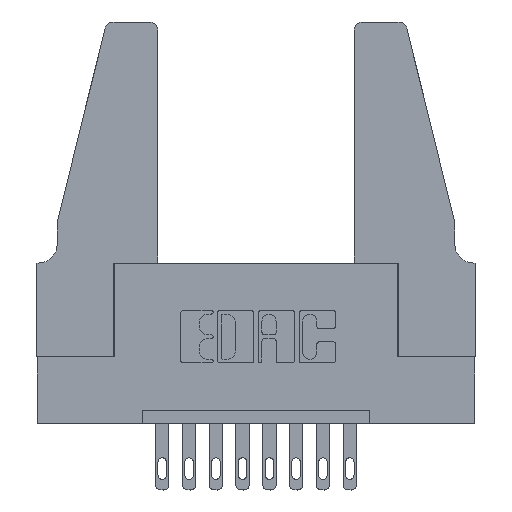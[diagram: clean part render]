
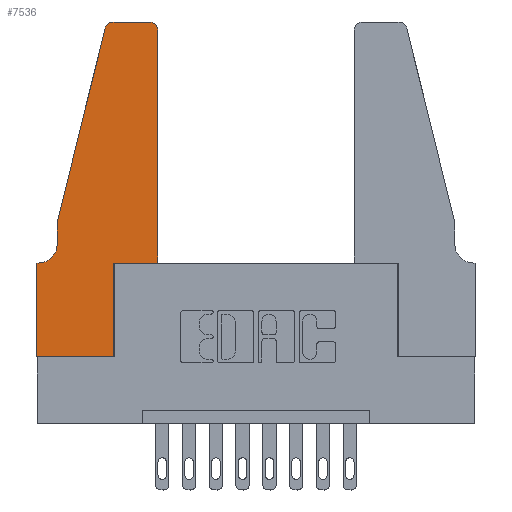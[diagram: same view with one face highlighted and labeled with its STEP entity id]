
A CAD part, top view. The second image highlights one B-rep face of the part: STEP entity #7536.
In plain terms, the highlighted planar face has unit normal (0, 0, 1).
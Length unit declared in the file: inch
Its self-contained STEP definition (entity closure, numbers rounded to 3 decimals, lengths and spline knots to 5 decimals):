
#288 = ORIENTED_EDGE ( 'NONE', *, *, #12328, .T. ) ;
#302 = ORIENTED_EDGE ( 'NONE', *, *, #5168, .T. ) ;
#349 = CARTESIAN_POINT ( 'NONE',  ( 0., 0., 0.37 ) ) ;
#369 = VERTEX_POINT ( 'NONE', #10503 ) ;
#376 = VERTEX_POINT ( 'NONE', #10540 ) ;
#685 = CARTESIAN_POINT ( 'NONE',  ( 0.284, 1.25, 0.37 ) ) ;
#722 = CARTESIAN_POINT ( 'NONE',  ( 0.0055, 0.35, 0.37 ) ) ;
#741 = ORIENTED_EDGE ( 'NONE', *, *, #765, .T. ) ;
#765 = EDGE_CURVE ( 'NONE', #5627, #7048, #4184, .T. ) ;
#915 = VERTEX_POINT ( 'NONE', #685 ) ;
#920 = ORIENTED_EDGE ( 'NONE', *, *, #9803, .T. ) ;
#959 = DIRECTION ( 'NONE',  ( 0., -1., 0. ) ) ;
#1067 = VECTOR ( 'NONE', #7128, 39.37008 ) ;
#1470 = DIRECTION ( 'NONE',  ( 0., 1., 0. ) ) ;
#1717 = EDGE_CURVE ( 'NONE', #5296, #10723, #3999, .T. ) ;
#1803 = EDGE_CURVE ( 'NONE', #6088, #8134, #10156, .T. ) ;
#2333 = DIRECTION ( 'NONE',  ( -1., 0., 0. ) ) ;
#2609 = DIRECTION ( 'NONE',  ( 0., 0., 1. ) ) ;
#2807 = CARTESIAN_POINT ( 'NONE',  ( 0.4505, 0.35, 0.37 ) ) ;
#2859 = DIRECTION ( 'NONE',  ( 0., 0., -1. ) ) ;
#2982 = LINE ( 'NONE', #11435, #12341 ) ;
#3111 = AXIS2_PLACEMENT_3D ( 'NONE', #8343, #9375, #3386 ) ;
#3386 = DIRECTION ( 'NONE',  ( 1., 0., 0. ) ) ;
#3447 = EDGE_CURVE ( 'NONE', #369, #5296, #9225, .T. ) ;
#3465 = EDGE_CURVE ( 'NONE', #9035, #369, #9377, .T. ) ;
#3548 = ORIENTED_EDGE ( 'NONE', *, *, #1803, .T. ) ;
#3670 = DIRECTION ( 'NONE',  ( 1., 0., 0. ) ) ;
#3714 = DIRECTION ( 'NONE',  ( 0., 0., 1. ) ) ;
#3924 = ORIENTED_EDGE ( 'NONE', *, *, #3465, .T. ) ;
#3981 = CARTESIAN_POINT ( 'NONE',  ( 0.4505, 0.35, 0.37 ) ) ;
#3999 = LINE ( 'NONE', #349, #1067 ) ;
#4130 = ORIENTED_EDGE ( 'NONE', *, *, #12606, .T. ) ;
#4184 = LINE ( 'NONE', #6381, #11858 ) ;
#4305 = CARTESIAN_POINT ( 'NONE',  ( 0., 0., 0.37 ) ) ;
#4671 = ORIENTED_EDGE ( 'NONE', *, *, #7869, .T. ) ;
#4696 = CARTESIAN_POINT ( 'NONE',  ( 0., 0.35, 0.37 ) ) ;
#4741 = CIRCLE ( 'NONE', #12590, 0.03 ) ;
#5082 = CARTESIAN_POINT ( 'NONE',  ( 0.4205, 1.25, 0.37 ) ) ;
#5121 = AXIS2_PLACEMENT_3D ( 'NONE', #6804, #2859, #10729 ) ;
#5148 = CARTESIAN_POINT ( 'NONE',  ( 0.0755, 0.5, 0.37 ) ) ;
#5168 = EDGE_CURVE ( 'NONE', #915, #6088, #8105, .T. ) ;
#5272 = CARTESIAN_POINT ( 'NONE',  ( 0.0755, 0.35, 0.37 ) ) ;
#5296 = VERTEX_POINT ( 'NONE', #4305 ) ;
#5300 = VECTOR ( 'NONE', #10256, 39.37008 ) ;
#5401 = CARTESIAN_POINT ( 'NONE',  ( 0.25487, 1.22718, 0.37 ) ) ;
#5627 = VERTEX_POINT ( 'NONE', #3981 ) ;
#5634 = VECTOR ( 'NONE', #8939, 39.37008 ) ;
#5781 = ORIENTED_EDGE ( 'NONE', *, *, #3447, .T. ) ;
#5830 = VECTOR ( 'NONE', #9705, 39.37008 ) ;
#5879 = CARTESIAN_POINT ( 'NONE',  ( 0.4505, 1.22, 0.37 ) ) ;
#6088 = VERTEX_POINT ( 'NONE', #5401 ) ;
#6095 = CARTESIAN_POINT ( 'NONE',  ( 0.0755, 0.5, 0.37 ) ) ;
#6145 = EDGE_CURVE ( 'NONE', #9045, #915, #10532, .T. ) ;
#6301 = CARTESIAN_POINT ( 'NONE',  ( 0.2605, 1.25, 0.37 ) ) ;
#6381 = CARTESIAN_POINT ( 'NONE',  ( 0.4505, 0.35, 0.37 ) ) ;
#6804 = CARTESIAN_POINT ( 'NONE',  ( 0.0055, 0.42, 0.37 ) ) ;
#7048 = VERTEX_POINT ( 'NONE', #5879 ) ;
#7128 = DIRECTION ( 'NONE',  ( 1., 0., 0. ) ) ;
#7437 = DIRECTION ( 'NONE',  ( 0., 1., 0. ) ) ;
#7446 = CARTESIAN_POINT ( 'NONE',  ( 0.0755, 0.42, 0.37 ) ) ;
#7512 = CARTESIAN_POINT ( 'NONE',  ( 0.4205, 1.22, 0.37 ) ) ;
#7536 = ADVANCED_FACE ( 'NONE', ( #8043 ), #8731, .T. ) ;
#7869 = EDGE_CURVE ( 'NONE', #8909, #9035, #11257, .T. ) ;
#7997 = LINE ( 'NONE', #2807, #5830 ) ;
#8043 = FACE_OUTER_BOUND ( 'NONE', #9837, .T. ) ;
#8105 = CIRCLE ( 'NONE', #3111, 0.03 ) ;
#8134 = VERTEX_POINT ( 'NONE', #11085 ) ;
#8163 = VECTOR ( 'NONE', #11046, 39.37008 ) ;
#8239 = LINE ( 'NONE', #5148, #5634 ) ;
#8343 = CARTESIAN_POINT ( 'NONE',  ( 0.284, 1.22, 0.37 ) ) ;
#8731 = PLANE ( 'NONE',  #10475 ) ;
#8909 = VERTEX_POINT ( 'NONE', #7446 ) ;
#8939 = DIRECTION ( 'NONE',  ( 0., -1., 0. ) ) ;
#9035 = VERTEX_POINT ( 'NONE', #722 ) ;
#9045 = VERTEX_POINT ( 'NONE', #5082 ) ;
#9075 = VECTOR ( 'NONE', #2333, 39.37008 ) ;
#9225 = LINE ( 'NONE', #9922, #12406 ) ;
#9375 = DIRECTION ( 'NONE',  ( 0., 0., 1. ) ) ;
#9377 = LINE ( 'NONE', #5272, #9075 ) ;
#9705 = DIRECTION ( 'NONE',  ( 1., 0., 0. ) ) ;
#9803 = EDGE_CURVE ( 'NONE', #376, #5627, #7997, .T. ) ;
#9837 = EDGE_LOOP ( 'NONE', ( #10864, #302, #3548, #288, #4671, #3924, #5781, #12281, #4130, #920, #741, #10153 ) ) ;
#9887 = EDGE_CURVE ( 'NONE', #7048, #9045, #4741, .T. ) ;
#9922 = CARTESIAN_POINT ( 'NONE',  ( 0., 0., 0.37 ) ) ;
#10153 = ORIENTED_EDGE ( 'NONE', *, *, #9887, .T. ) ;
#10156 = LINE ( 'NONE', #6095, #8163 ) ;
#10256 = DIRECTION ( 'NONE',  ( -1., 0., 0. ) ) ;
#10475 = AXIS2_PLACEMENT_3D ( 'NONE', #4696, #3714, #12651 ) ;
#10503 = CARTESIAN_POINT ( 'NONE',  ( 0., 0.35, 0.37 ) ) ;
#10532 = LINE ( 'NONE', #6301, #5300 ) ;
#10540 = CARTESIAN_POINT ( 'NONE',  ( 0.2865, 0.35, 0.37 ) ) ;
#10723 = VERTEX_POINT ( 'NONE', #12193 ) ;
#10729 = DIRECTION ( 'NONE',  ( -1., 0., 0. ) ) ;
#10864 = ORIENTED_EDGE ( 'NONE', *, *, #6145, .T. ) ;
#11046 = DIRECTION ( 'NONE',  ( -0.239, -0.971, 0. ) ) ;
#11085 = CARTESIAN_POINT ( 'NONE',  ( 0.0755, 0.5, 0.37 ) ) ;
#11257 = CIRCLE ( 'NONE', #5121, 0.07 ) ;
#11435 = CARTESIAN_POINT ( 'NONE',  ( 0.2865, 0.35, 0.37 ) ) ;
#11858 = VECTOR ( 'NONE', #1470, 39.37008 ) ;
#12193 = CARTESIAN_POINT ( 'NONE',  ( 0.2865, 0., 0.37 ) ) ;
#12281 = ORIENTED_EDGE ( 'NONE', *, *, #1717, .T. ) ;
#12328 = EDGE_CURVE ( 'NONE', #8134, #8909, #8239, .T. ) ;
#12341 = VECTOR ( 'NONE', #7437, 39.37008 ) ;
#12406 = VECTOR ( 'NONE', #959, 39.37008 ) ;
#12590 = AXIS2_PLACEMENT_3D ( 'NONE', #7512, #2609, #3670 ) ;
#12606 = EDGE_CURVE ( 'NONE', #10723, #376, #2982, .T. ) ;
#12651 = DIRECTION ( 'NONE',  ( 1., 0., 0. ) ) ;
